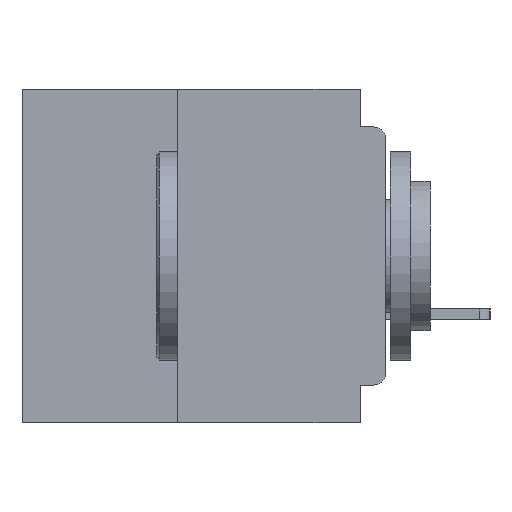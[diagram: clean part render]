
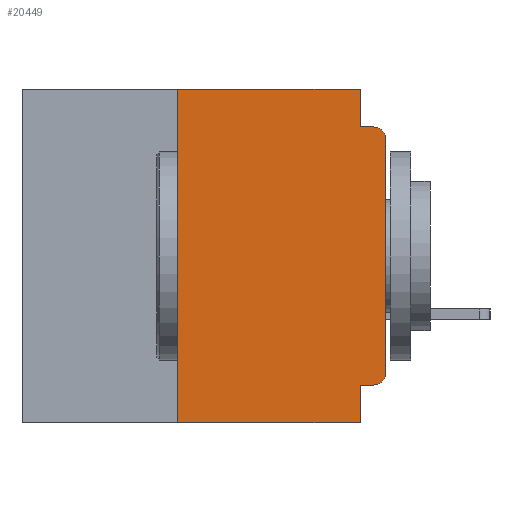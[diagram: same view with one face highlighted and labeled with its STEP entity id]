
A CAD part, left-side view. The second image highlights one B-rep face of the part: STEP entity #20449.
In plain terms, the highlighted planar face has unit normal (-1, 0, 0).
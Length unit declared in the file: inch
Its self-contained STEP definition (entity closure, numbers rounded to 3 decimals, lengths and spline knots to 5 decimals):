
#103 = DIRECTION ( 'NONE',  ( 1., 0., 0. ) ) ;
#161 = LINE ( 'NONE', #37880, #32918 ) ;
#232 = ORIENTED_EDGE ( 'NONE', *, *, #8924, .T. ) ;
#325 = CARTESIAN_POINT ( 'NONE',  ( 0., 0., -0.06 ) ) ;
#342 = DIRECTION ( 'NONE',  ( 0., 0., 1. ) ) ;
#517 = DIRECTION ( 'NONE',  ( 0., 0., -1. ) ) ;
#889 = CARTESIAN_POINT ( 'NONE',  ( 0., 0.25, -0.4 ) ) ;
#1212 = LINE ( 'NONE', #16160, #25595 ) ;
#1490 = CARTESIAN_POINT ( 'NONE',  ( 0., 0.031, 0. ) ) ;
#2087 = LINE ( 'NONE', #23034, #16979 ) ;
#2360 = DIRECTION ( 'NONE',  ( -1., 0., 0. ) ) ;
#2704 = AXIS2_PLACEMENT_3D ( 'NONE', #21412, #2360, #24602 ) ;
#3027 = ORIENTED_EDGE ( 'NONE', *, *, #15300, .F. ) ;
#4449 = VERTEX_POINT ( 'NONE', #33473 ) ;
#4578 = CARTESIAN_POINT ( 'NONE',  ( 0., 0.25, -0.4 ) ) ;
#4786 = DIRECTION ( 'NONE',  ( 0., -1., 0. ) ) ;
#5031 = LINE ( 'NONE', #1490, #30355 ) ;
#5198 = CARTESIAN_POINT ( 'NONE',  ( 0., 0.031, -0.4 ) ) ;
#7528 = CIRCLE ( 'NONE', #2704, 0.015 ) ;
#8471 = EDGE_CURVE ( 'NONE', #13900, #31075, #22861, .T. ) ;
#8728 = EDGE_CURVE ( 'NONE', #38396, #35413, #21344, .T. ) ;
#8924 = EDGE_CURVE ( 'NONE', #12927, #26216, #38645, .T. ) ;
#9487 = ORIENTED_EDGE ( 'NONE', *, *, #24830, .T. ) ;
#9558 = CARTESIAN_POINT ( 'NONE',  ( 0., 0.437, 0. ) ) ;
#10176 = ORIENTED_EDGE ( 'NONE', *, *, #8728, .F. ) ;
#12594 = EDGE_CURVE ( 'NONE', #35413, #12656, #19053, .T. ) ;
#12652 = CARTESIAN_POINT ( 'NONE',  ( 0., 0., -0.34 ) ) ;
#12656 = VERTEX_POINT ( 'NONE', #5198 ) ;
#12927 = VERTEX_POINT ( 'NONE', #325 ) ;
#13900 = VERTEX_POINT ( 'NONE', #889 ) ;
#14801 = VECTOR ( 'NONE', #4786, 39.37008 ) ;
#15300 = EDGE_CURVE ( 'NONE', #31075, #38332, #31713, .T. ) ;
#16160 = CARTESIAN_POINT ( 'NONE',  ( 0., 0., 0. ) ) ;
#16384 = EDGE_LOOP ( 'NONE', ( #28398, #232, #40061, #17288, #3027, #16847, #9487, #21737, #10176, #33479 ) ) ;
#16847 = ORIENTED_EDGE ( 'NONE', *, *, #8471, .F. ) ;
#16979 = VECTOR ( 'NONE', #38922, 39.37008 ) ;
#17288 = ORIENTED_EDGE ( 'NONE', *, *, #25748, .F. ) ;
#18615 = FACE_OUTER_BOUND ( 'NONE', #16384, .T. ) ;
#19053 = LINE ( 'NONE', #20786, #33901 ) ;
#19566 = DIRECTION ( 'NONE',  ( -1., 0., 0. ) ) ;
#20420 = CARTESIAN_POINT ( 'NONE',  ( 0., 0.031, 0. ) ) ;
#20430 = DIRECTION ( 'NONE',  ( 0., 0., 1. ) ) ;
#20449 = ADVANCED_FACE ( 'NONE', ( #18615 ), #31766, .F. ) ;
#20786 = CARTESIAN_POINT ( 'NONE',  ( 0., 0.031, -0.4 ) ) ;
#21344 = LINE ( 'NONE', #34389, #37181 ) ;
#21412 = CARTESIAN_POINT ( 'NONE',  ( 0., 0.015, -0.34 ) ) ;
#21737 = ORIENTED_EDGE ( 'NONE', *, *, #12594, .F. ) ;
#22028 = EDGE_CURVE ( 'NONE', #38396, #36301, #7528, .T. ) ;
#22371 = DIRECTION ( 'NONE',  ( 0., 0., -1. ) ) ;
#22723 = CARTESIAN_POINT ( 'NONE',  ( 0., 0.015, -0.045 ) ) ;
#22861 = LINE ( 'NONE', #4578, #38687 ) ;
#23034 = CARTESIAN_POINT ( 'NONE',  ( 0., 0.437, -0.4 ) ) ;
#23729 = DIRECTION ( 'NONE',  ( 0., 0., -1. ) ) ;
#23871 = CARTESIAN_POINT ( 'NONE',  ( 0., 0.437, 0. ) ) ;
#23981 = EDGE_CURVE ( 'NONE', #4449, #26216, #161, .T. ) ;
#24506 = AXIS2_PLACEMENT_3D ( 'NONE', #9558, #103, #22371 ) ;
#24577 = AXIS2_PLACEMENT_3D ( 'NONE', #38522, #19566, #517 ) ;
#24602 = DIRECTION ( 'NONE',  ( 0., 0., -1. ) ) ;
#24705 = CARTESIAN_POINT ( 'NONE',  ( 0., 0.25, 0. ) ) ;
#24830 = EDGE_CURVE ( 'NONE', #13900, #12656, #2087, .T. ) ;
#25322 = DIRECTION ( 'NONE',  ( 0., -1., 0. ) ) ;
#25595 = VECTOR ( 'NONE', #342, 39.37008 ) ;
#25748 = EDGE_CURVE ( 'NONE', #38332, #4449, #5031, .T. ) ;
#26216 = VERTEX_POINT ( 'NONE', #22723 ) ;
#28398 = ORIENTED_EDGE ( 'NONE', *, *, #29422, .T. ) ;
#29422 = EDGE_CURVE ( 'NONE', #36301, #12927, #1212, .T. ) ;
#30355 = VECTOR ( 'NONE', #23729, 39.37008 ) ;
#31075 = VERTEX_POINT ( 'NONE', #24705 ) ;
#31713 = LINE ( 'NONE', #23871, #14801 ) ;
#31766 = PLANE ( 'NONE',  #24506 ) ;
#32918 = VECTOR ( 'NONE', #25322, 39.37008 ) ;
#33405 = CARTESIAN_POINT ( 'NONE',  ( 0., 0.015, -0.355 ) ) ;
#33473 = CARTESIAN_POINT ( 'NONE',  ( 0., 0.031, -0.045 ) ) ;
#33479 = ORIENTED_EDGE ( 'NONE', *, *, #22028, .T. ) ;
#33901 = VECTOR ( 'NONE', #36692, 39.37008 ) ;
#33915 = CARTESIAN_POINT ( 'NONE',  ( 0., 0.031, -0.355 ) ) ;
#34389 = CARTESIAN_POINT ( 'NONE',  ( 0., 0., -0.355 ) ) ;
#35413 = VERTEX_POINT ( 'NONE', #33915 ) ;
#36301 = VERTEX_POINT ( 'NONE', #12652 ) ;
#36692 = DIRECTION ( 'NONE',  ( 0., 0., -1. ) ) ;
#37181 = VECTOR ( 'NONE', #37437, 39.37008 ) ;
#37437 = DIRECTION ( 'NONE',  ( 0., 1., 0. ) ) ;
#37880 = CARTESIAN_POINT ( 'NONE',  ( 0., 0., -0.045 ) ) ;
#38332 = VERTEX_POINT ( 'NONE', #20420 ) ;
#38396 = VERTEX_POINT ( 'NONE', #33405 ) ;
#38522 = CARTESIAN_POINT ( 'NONE',  ( 0., 0.015, -0.06 ) ) ;
#38645 = CIRCLE ( 'NONE', #24577, 0.015 ) ;
#38687 = VECTOR ( 'NONE', #20430, 39.37008 ) ;
#38922 = DIRECTION ( 'NONE',  ( 0., -1., 0. ) ) ;
#40061 = ORIENTED_EDGE ( 'NONE', *, *, #23981, .F. ) ;
